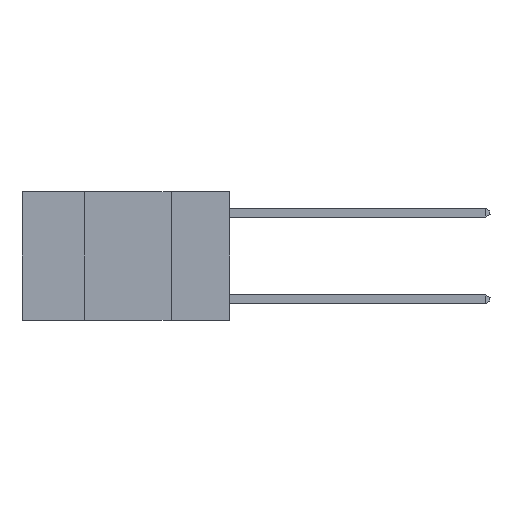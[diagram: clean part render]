
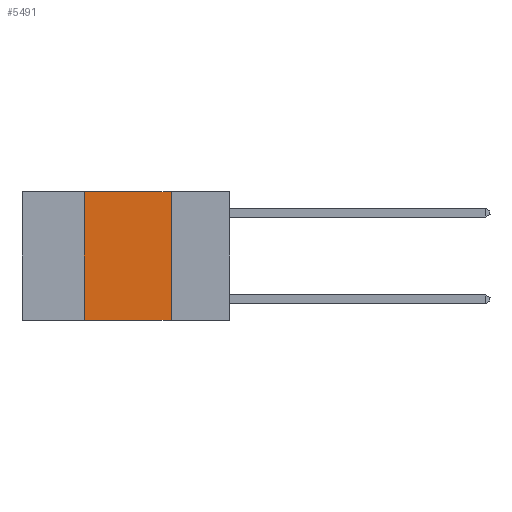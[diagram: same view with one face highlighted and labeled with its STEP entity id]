
A CAD part, left-side view. The second image highlights one B-rep face of the part: STEP entity #5491.
In plain terms, the highlighted planar face has unit normal (-1, 0, 0).
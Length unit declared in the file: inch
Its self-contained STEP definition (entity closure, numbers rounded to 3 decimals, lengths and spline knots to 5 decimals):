
#347 = CARTESIAN_POINT ( 'NONE',  ( 0., 0.42, 0. ) ) ;
#436 = CARTESIAN_POINT ( 'NONE',  ( 0., 0.17, 0. ) ) ;
#504 = VERTEX_POINT ( 'NONE', #436 ) ;
#1386 = CARTESIAN_POINT ( 'NONE',  ( 0., 0.42, -0.37 ) ) ;
#1699 = DIRECTION ( 'NONE',  ( 1., 0., 0. ) ) ;
#2194 = VERTEX_POINT ( 'NONE', #1386 ) ;
#2687 = DIRECTION ( 'NONE',  ( 0., 0., 1. ) ) ;
#2730 = ORIENTED_EDGE ( 'NONE', *, *, #11227, .F. ) ;
#3530 = LINE ( 'NONE', #8343, #5566 ) ;
#3634 = EDGE_CURVE ( 'NONE', #2194, #7359, #13635, .T. ) ;
#4449 = LINE ( 'NONE', #6931, #7635 ) ;
#4496 = CARTESIAN_POINT ( 'NONE',  ( 0., 0.17, 0. ) ) ;
#4695 = DIRECTION ( 'NONE',  ( 0., -1., 0. ) ) ;
#4816 = DIRECTION ( 'NONE',  ( 0., -1., 0. ) ) ;
#5491 = ADVANCED_FACE ( 'NONE', ( #15091 ), #6518, .F. ) ;
#5566 = VECTOR ( 'NONE', #4816, 39.37008 ) ;
#5862 = DIRECTION ( 'NONE',  ( 0., 0., -1. ) ) ;
#6518 = PLANE ( 'NONE',  #15529 ) ;
#6647 = ORIENTED_EDGE ( 'NONE', *, *, #13416, .T. ) ;
#6674 = ORIENTED_EDGE ( 'NONE', *, *, #9325, .F. ) ;
#6931 = CARTESIAN_POINT ( 'NONE',  ( 0., 0.6, -0.37 ) ) ;
#7136 = VECTOR ( 'NONE', #5862, 39.37008 ) ;
#7359 = VERTEX_POINT ( 'NONE', #7864 ) ;
#7635 = VECTOR ( 'NONE', #4695, 39.37008 ) ;
#7802 = DIRECTION ( 'NONE',  ( 0., 0., -1. ) ) ;
#7864 = CARTESIAN_POINT ( 'NONE',  ( 0., 0.42, 0. ) ) ;
#8079 = ORIENTED_EDGE ( 'NONE', *, *, #3634, .F. ) ;
#8343 = CARTESIAN_POINT ( 'NONE',  ( 0., 0.6, 0. ) ) ;
#9325 = EDGE_CURVE ( 'NONE', #504, #14404, #14350, .T. ) ;
#11227 = EDGE_CURVE ( 'NONE', #7359, #504, #3530, .T. ) ;
#11332 = CARTESIAN_POINT ( 'NONE',  ( 0., 0.6, 0. ) ) ;
#11337 = CARTESIAN_POINT ( 'NONE',  ( 0., 0.17, -0.37 ) ) ;
#13416 = EDGE_CURVE ( 'NONE', #2194, #14404, #4449, .T. ) ;
#13635 = LINE ( 'NONE', #347, #15189 ) ;
#14350 = LINE ( 'NONE', #4496, #7136 ) ;
#14404 = VERTEX_POINT ( 'NONE', #11337 ) ;
#15091 = FACE_OUTER_BOUND ( 'NONE', #15275, .T. ) ;
#15189 = VECTOR ( 'NONE', #2687, 39.37008 ) ;
#15275 = EDGE_LOOP ( 'NONE', ( #6674, #2730, #8079, #6647 ) ) ;
#15529 = AXIS2_PLACEMENT_3D ( 'NONE', #11332, #1699, #7802 ) ;
